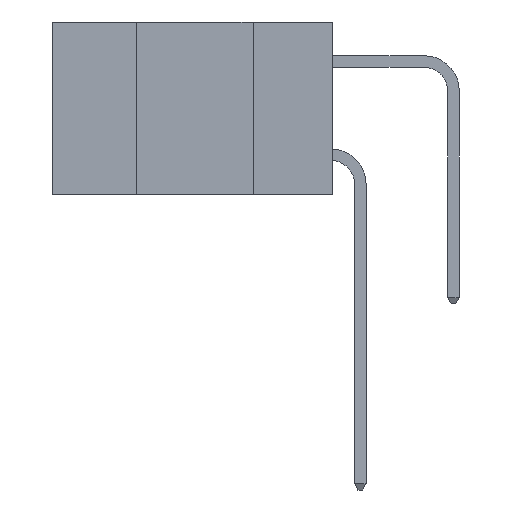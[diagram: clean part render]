
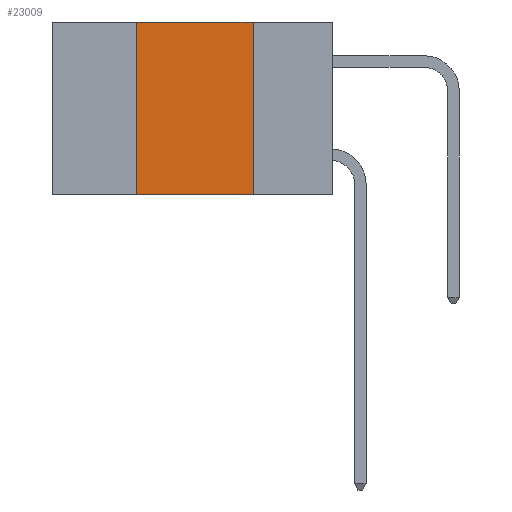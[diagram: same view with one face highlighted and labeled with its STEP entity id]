
A CAD part, left-side view. The second image highlights one B-rep face of the part: STEP entity #23009.
In plain terms, the highlighted planar face has unit normal (-1, 0, 0).
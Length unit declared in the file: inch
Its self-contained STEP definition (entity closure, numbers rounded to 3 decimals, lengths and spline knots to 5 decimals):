
#280 = LINE ( 'NONE', #5159, #16303 ) ;
#1956 = CARTESIAN_POINT ( 'NONE',  ( 0., 0.42, -0.37 ) ) ;
#2213 = AXIS2_PLACEMENT_3D ( 'NONE', #24982, #5135, #19063 ) ;
#2747 = LINE ( 'NONE', #5897, #13426 ) ;
#3100 = PLANE ( 'NONE',  #2213 ) ;
#4711 = CARTESIAN_POINT ( 'NONE',  ( 0., 0.17, -0.37 ) ) ;
#5135 = DIRECTION ( 'NONE',  ( 1., 0., 0. ) ) ;
#5159 = CARTESIAN_POINT ( 'NONE',  ( 0., 0.42, -0.37 ) ) ;
#5323 = CARTESIAN_POINT ( 'NONE',  ( 0., 0.6, -0.37 ) ) ;
#5375 = EDGE_CURVE ( 'NONE', #11088, #24917, #5895, .T. ) ;
#5895 = LINE ( 'NONE', #18777, #10632 ) ;
#5897 = CARTESIAN_POINT ( 'NONE',  ( 0., 0.17, -0.37 ) ) ;
#6531 = VERTEX_POINT ( 'NONE', #1956 ) ;
#8626 = VERTEX_POINT ( 'NONE', #4711 ) ;
#8815 = CARTESIAN_POINT ( 'NONE',  ( 0., 0.42, 0. ) ) ;
#10632 = VECTOR ( 'NONE', #16788, 39.37008 ) ;
#11088 = VERTEX_POINT ( 'NONE', #8815 ) ;
#11410 = DIRECTION ( 'NONE',  ( 0., -1., 0. ) ) ;
#13231 = ORIENTED_EDGE ( 'NONE', *, *, #24075, .T. ) ;
#13426 = VECTOR ( 'NONE', #19813, 39.37008 ) ;
#14130 = CARTESIAN_POINT ( 'NONE',  ( 0., 0.17, 0. ) ) ;
#14820 = VECTOR ( 'NONE', #11410, 39.37008 ) ;
#14830 = EDGE_LOOP ( 'NONE', ( #19796, #25073, #19426, #13231 ) ) ;
#15189 = FACE_OUTER_BOUND ( 'NONE', #14830, .T. ) ;
#16303 = VECTOR ( 'NONE', #21130, 39.37008 ) ;
#16788 = DIRECTION ( 'NONE',  ( 0., -1., 0. ) ) ;
#16904 = EDGE_CURVE ( 'NONE', #6531, #11088, #280, .T. ) ;
#18573 = EDGE_CURVE ( 'NONE', #24917, #8626, #2747, .T. ) ;
#18777 = CARTESIAN_POINT ( 'NONE',  ( 0., 0.6, 0. ) ) ;
#19063 = DIRECTION ( 'NONE',  ( 0., 0., -1. ) ) ;
#19426 = ORIENTED_EDGE ( 'NONE', *, *, #16904, .F. ) ;
#19796 = ORIENTED_EDGE ( 'NONE', *, *, #18573, .F. ) ;
#19813 = DIRECTION ( 'NONE',  ( 0., 0., -1. ) ) ;
#21130 = DIRECTION ( 'NONE',  ( 0., 0., 1. ) ) ;
#23009 = ADVANCED_FACE ( 'NONE', ( #15189 ), #3100, .F. ) ;
#24075 = EDGE_CURVE ( 'NONE', #6531, #8626, #25383, .T. ) ;
#24917 = VERTEX_POINT ( 'NONE', #14130 ) ;
#24982 = CARTESIAN_POINT ( 'NONE',  ( 0., 0.6, 0. ) ) ;
#25073 = ORIENTED_EDGE ( 'NONE', *, *, #5375, .F. ) ;
#25383 = LINE ( 'NONE', #5323, #14820 ) ;
